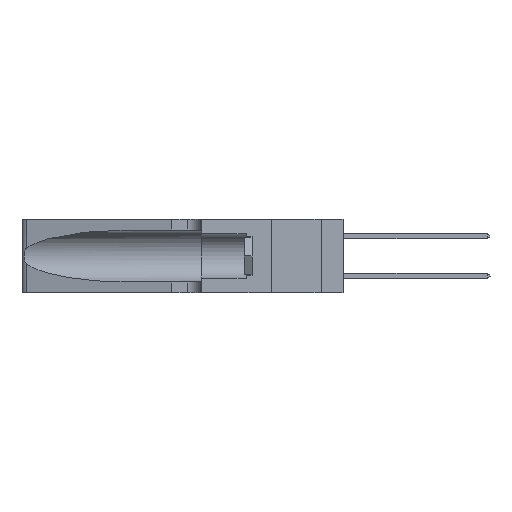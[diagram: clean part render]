
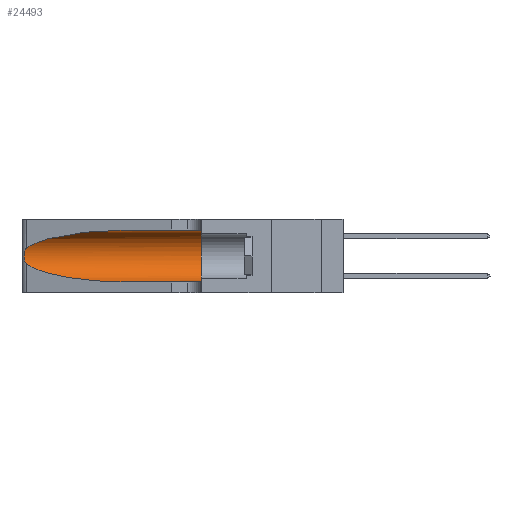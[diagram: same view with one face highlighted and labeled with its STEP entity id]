
A CAD part, left-side view. The second image highlights one B-rep face of the part: STEP entity #24493.
In plain terms, the highlighted cylindrical face has radius 3.308 mm (diameter 6.617 mm), a partial arc.
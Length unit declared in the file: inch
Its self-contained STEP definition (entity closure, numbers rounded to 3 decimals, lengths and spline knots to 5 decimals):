
#301 = VERTEX_POINT ( 'NONE', #24122 ) ;
#304 = DIRECTION ( 'NONE',  ( 0., -1., 0. ) ) ;
#967 = CARTESIAN_POINT ( 'NONE',  ( 0.25487, 1.22718, 0.14631 ) ) ;
#1067 = EDGE_CURVE ( 'NONE', #24241, #33434, #15019, .T. ) ;
#2779 = CARTESIAN_POINT ( 'NONE',  ( 0.1305, 0.72297, 0.31525 ) ) ;
#2907 = VERTEX_POINT ( 'NONE', #12532 ) ;
#3527 = CARTESIAN_POINT ( 'NONE',  ( 0.25787, 1.23484, 0.2124 ) ) ;
#5306 = CARTESIAN_POINT ( 'NONE',  ( 0.25789, 1.23486, 0.15765 ) ) ;
#5343 = LINE ( 'NONE', #34642, #40484 ) ;
#5743 = DIRECTION ( 'NONE',  ( 0., 0., 1. ) ) ;
#5785 = CARTESIAN_POINT ( 'NONE',  ( 0.2373, 1.15595, 0.28018 ) ) ;
#8108 = EDGE_LOOP ( 'NONE', ( #24996, #34315, #32350, #43528, #29756, #29176 ) ) ;
#8997 =( BOUNDED_CURVE ( )  B_SPLINE_CURVE ( 3, ( #26184, #36310, #5785, #9419 ),
 .UNSPECIFIED., .F., .T. ) 
 B_SPLINE_CURVE_WITH_KNOTS ( ( 4, 4 ),
 ( 1.5708, 2.84003 ),
 .UNSPECIFIED. ) 
 CURVE ( )  GEOMETRIC_REPRESENTATION_ITEM ( )  RATIONAL_B_SPLINE_CURVE ( ( 1., 0.87, 0.87, 1. ) ) 
 REPRESENTATION_ITEM ( '' )  );
#9419 = CARTESIAN_POINT ( 'NONE',  ( 0.25487, 1.22718, 0.22369 ) ) ;
#12532 = CARTESIAN_POINT ( 'NONE',  ( 0.1305, 0.35, 0.31525 ) ) ;
#14207 =( BOUNDED_CURVE ( )  B_SPLINE_CURVE ( 3, ( #20364, #26162, #29512, #29381 ),
 .UNSPECIFIED., .F., .F. ) 
 B_SPLINE_CURVE_WITH_KNOTS ( ( 4, 4 ),
 ( 3.44316, 4.71239 ),
 .UNSPECIFIED. ) 
 CURVE ( )  GEOMETRIC_REPRESENTATION_ITEM ( )  RATIONAL_B_SPLINE_CURVE ( ( 1., 0.87, 0.87, 1. ) ) 
 REPRESENTATION_ITEM ( '' )  );
#14882 = FACE_OUTER_BOUND ( 'NONE', #8108, .T. ) ;
#15019 = B_SPLINE_CURVE_WITH_KNOTS ( 'NONE', 3,
 ( #34803, #36969, #20513, #3527, #26066, #38814, #24753, #20363, #20695, #39060, #5306, #38302, #38003, #967 ),
 .UNSPECIFIED., .F., .F.,
 ( 4, 2, 2, 2, 2, 2, 4 ),
 ( 0., 0.00027, 0.00053, 0.00107, 0.0016, 0.00187, 0.00214 ),
 .UNSPECIFIED. ) ;
#16265 = CARTESIAN_POINT ( 'NONE',  ( 0.1305, 1.61858, 0.05475 ) ) ;
#18342 = DIRECTION ( 'NONE',  ( 0., -1., 0. ) ) ;
#18521 = AXIS2_PLACEMENT_3D ( 'NONE', #38473, #18342, #18777 ) ;
#18777 = DIRECTION ( 'NONE',  ( 0., 0., -1. ) ) ;
#18834 = EDGE_CURVE ( 'NONE', #33434, #29732, #14207, .T. ) ;
#19049 = DIRECTION ( 'NONE',  ( 0., 1., 0. ) ) ;
#19941 = CARTESIAN_POINT ( 'NONE',  ( 0.25487, 1.22718, 0.14631 ) ) ;
#20363 = CARTESIAN_POINT ( 'NONE',  ( 0.26075, 1.23896, 0.178 ) ) ;
#20364 = CARTESIAN_POINT ( 'NONE',  ( 0.25487, 1.22718, 0.14631 ) ) ;
#20513 = CARTESIAN_POINT ( 'NONE',  ( 0.25639, 1.23184, 0.21858 ) ) ;
#20695 = CARTESIAN_POINT ( 'NONE',  ( 0.26017, 1.23833, 0.17102 ) ) ;
#23471 = CARTESIAN_POINT ( 'NONE',  ( 0.25487, 1.22718, 0.22369 ) ) ;
#24122 = CARTESIAN_POINT ( 'NONE',  ( 0.1305, 0.35, 0.05475 ) ) ;
#24241 = VERTEX_POINT ( 'NONE', #23471 ) ;
#24493 = ADVANCED_FACE ( 'NONE', ( #14882 ), #37920, .F. ) ;
#24532 = DIRECTION ( 'NONE',  ( 0., -1., 0. ) ) ;
#24753 = CARTESIAN_POINT ( 'NONE',  ( 0.26075, 1.23896, 0.19203 ) ) ;
#24996 = ORIENTED_EDGE ( 'NONE', *, *, #33347, .T. ) ;
#25168 = EDGE_CURVE ( 'NONE', #35957, #2907, #5343, .T. ) ;
#25728 = CARTESIAN_POINT ( 'NONE',  ( 0.1305, 0.35, 0.185 ) ) ;
#26066 = CARTESIAN_POINT ( 'NONE',  ( 0.25854, 1.2359, 0.20912 ) ) ;
#26162 = CARTESIAN_POINT ( 'NONE',  ( 0.2373, 1.15595, 0.08982 ) ) ;
#26184 = CARTESIAN_POINT ( 'NONE',  ( 0.1305, 0.72297, 0.31525 ) ) ;
#27958 = EDGE_CURVE ( 'NONE', #29732, #301, #29269, .T. ) ;
#29176 = ORIENTED_EDGE ( 'NONE', *, *, #25168, .F. ) ;
#29269 = LINE ( 'NONE', #16265, #36102 ) ;
#29381 = CARTESIAN_POINT ( 'NONE',  ( 0.1305, 0.72297, 0.05475 ) ) ;
#29512 = CARTESIAN_POINT ( 'NONE',  ( 0.18966, 0.96281, 0.05475 ) ) ;
#29717 = CIRCLE ( 'NONE', #43463, 0.13025 ) ;
#29732 = VERTEX_POINT ( 'NONE', #30704 ) ;
#29756 = ORIENTED_EDGE ( 'NONE', *, *, #42535, .F. ) ;
#30704 = CARTESIAN_POINT ( 'NONE',  ( 0.1305, 0.72297, 0.05475 ) ) ;
#32350 = ORIENTED_EDGE ( 'NONE', *, *, #18834, .T. ) ;
#33347 = EDGE_CURVE ( 'NONE', #35957, #24241, #8997, .T. ) ;
#33434 = VERTEX_POINT ( 'NONE', #19941 ) ;
#34315 = ORIENTED_EDGE ( 'NONE', *, *, #1067, .T. ) ;
#34642 = CARTESIAN_POINT ( 'NONE',  ( 0.1305, 1.61858, 0.31525 ) ) ;
#34803 = CARTESIAN_POINT ( 'NONE',  ( 0.25487, 1.22718, 0.22369 ) ) ;
#35957 = VERTEX_POINT ( 'NONE', #2779 ) ;
#36102 = VECTOR ( 'NONE', #304, 39.37008 ) ;
#36310 = CARTESIAN_POINT ( 'NONE',  ( 0.18966, 0.96281, 0.31525 ) ) ;
#36969 = CARTESIAN_POINT ( 'NONE',  ( 0.25555, 1.22994, 0.2215 ) ) ;
#37920 = CYLINDRICAL_SURFACE ( 'NONE', #18521, 0.13025 ) ;
#38003 = CARTESIAN_POINT ( 'NONE',  ( 0.25555, 1.22993, 0.14849 ) ) ;
#38302 = CARTESIAN_POINT ( 'NONE',  ( 0.25639, 1.23186, 0.15144 ) ) ;
#38473 = CARTESIAN_POINT ( 'NONE',  ( 0.1305, 1.61858, 0.185 ) ) ;
#38814 = CARTESIAN_POINT ( 'NONE',  ( 0.26018, 1.23835, 0.19895 ) ) ;
#39060 = CARTESIAN_POINT ( 'NONE',  ( 0.25856, 1.23593, 0.16098 ) ) ;
#40484 = VECTOR ( 'NONE', #24532, 39.37008 ) ;
#42535 = EDGE_CURVE ( 'NONE', #2907, #301, #29717, .T. ) ;
#43463 = AXIS2_PLACEMENT_3D ( 'NONE', #25728, #19049, #5743 ) ;
#43528 = ORIENTED_EDGE ( 'NONE', *, *, #27958, .T. ) ;
